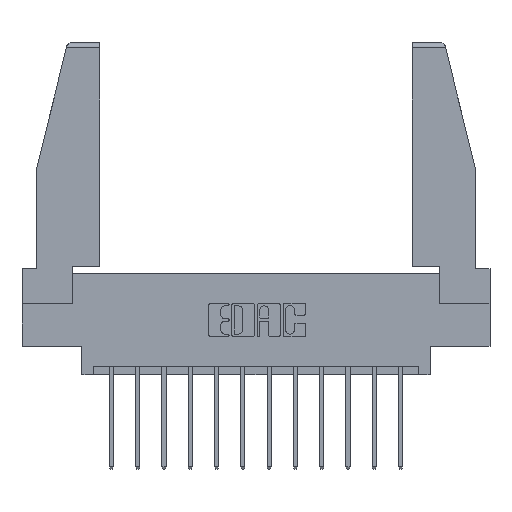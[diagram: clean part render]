
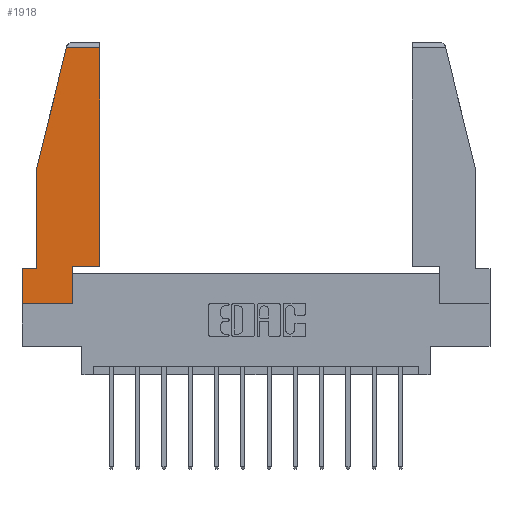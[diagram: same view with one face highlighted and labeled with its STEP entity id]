
A CAD part, top view. The second image highlights one B-rep face of the part: STEP entity #1918.
In plain terms, the highlighted planar face has unit normal (0, 0, 1).
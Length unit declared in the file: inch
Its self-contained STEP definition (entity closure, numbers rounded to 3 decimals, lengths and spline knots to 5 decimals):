
#11 = EDGE_CURVE ( 'NONE', #9317, #4856, #13222, .T. ) ;
#448 = VECTOR ( 'NONE', #8510, 39.37008 ) ;
#564 = VECTOR ( 'NONE', #9412, 39.37008 ) ;
#586 = DIRECTION ( 'NONE',  ( 1., 0., 0. ) ) ;
#639 = DIRECTION ( 'NONE',  ( 1., 0., 0. ) ) ;
#759 = CARTESIAN_POINT ( 'NONE',  ( 0., 1.52, 0. ) ) ;
#765 = VECTOR ( 'NONE', #3878, 39.37008 ) ;
#871 = ORIENTED_EDGE ( 'NONE', *, *, #11598, .T. ) ;
#887 = CARTESIAN_POINT ( 'NONE',  ( 0.297, 0., 0. ) ) ;
#981 = ORIENTED_EDGE ( 'NONE', *, *, #7468, .T. ) ;
#1092 = DIRECTION ( 'NONE',  ( 0., 1., 0. ) ) ;
#1780 = VECTOR ( 'NONE', #6536, 39.37008 ) ;
#1855 = LINE ( 'NONE', #9011, #7597 ) ;
#1918 = ADVANCED_FACE ( 'NONE', ( #15102 ), #10439, .T. ) ;
#2151 = LINE ( 'NONE', #12695, #1780 ) ;
#2437 = ORIENTED_EDGE ( 'NONE', *, *, #12441, .T. ) ;
#2641 = CARTESIAN_POINT ( 'NONE',  ( 0.086, 0.8, 0. ) ) ;
#2787 = VERTEX_POINT ( 'NONE', #12084 ) ;
#2929 = LINE ( 'NONE', #759, #448 ) ;
#3044 = CARTESIAN_POINT ( 'NONE',  ( 0.297, 0.223, 0. ) ) ;
#3161 = EDGE_CURVE ( 'NONE', #2787, #10127, #13903, .T. ) ;
#3176 = LINE ( 'NONE', #12828, #12902 ) ;
#3314 = VERTEX_POINT ( 'NONE', #3661 ) ;
#3504 = VERTEX_POINT ( 'NONE', #10144 ) ;
#3586 = EDGE_LOOP ( 'NONE', ( #15508, #981, #15374, #8361, #9837, #2437, #6179, #11562, #871 ) ) ;
#3661 = CARTESIAN_POINT ( 'NONE',  ( 0.086, 0.21, 0. ) ) ;
#3878 = DIRECTION ( 'NONE',  ( -0.239, -0.971, 0. ) ) ;
#3914 = CARTESIAN_POINT ( 'NONE',  ( 0.461, 0.223, 0. ) ) ;
#4030 = LINE ( 'NONE', #8741, #765 ) ;
#4105 = VERTEX_POINT ( 'NONE', #6369 ) ;
#4177 = EDGE_CURVE ( 'NONE', #4105, #3314, #7805, .T. ) ;
#4770 = CARTESIAN_POINT ( 'NONE',  ( 0.461, 0.223, 0. ) ) ;
#4856 = VERTEX_POINT ( 'NONE', #8624 ) ;
#6179 = ORIENTED_EDGE ( 'NONE', *, *, #12522, .T. ) ;
#6369 = CARTESIAN_POINT ( 'NONE',  ( 0.086, 0.8, 0. ) ) ;
#6416 = CARTESIAN_POINT ( 'NONE',  ( 0., 0., 0. ) ) ;
#6536 = DIRECTION ( 'NONE',  ( -1., 0., 0. ) ) ;
#7234 = VECTOR ( 'NONE', #639, 39.37008 ) ;
#7468 = EDGE_CURVE ( 'NONE', #4856, #12245, #2929, .T. ) ;
#7597 = VECTOR ( 'NONE', #586, 39.37008 ) ;
#7678 = EDGE_CURVE ( 'NONE', #3314, #3504, #2151, .T. ) ;
#7805 = LINE ( 'NONE', #2641, #15059 ) ;
#7808 = DIRECTION ( 'NONE',  ( 0., -1., 0. ) ) ;
#8361 = ORIENTED_EDGE ( 'NONE', *, *, #4177, .T. ) ;
#8510 = DIRECTION ( 'NONE',  ( -1., 0., 0. ) ) ;
#8624 = CARTESIAN_POINT ( 'NONE',  ( 0.461, 1.52, 0. ) ) ;
#8741 = CARTESIAN_POINT ( 'NONE',  ( 0.271, 1.55, 0. ) ) ;
#8818 = EDGE_CURVE ( 'NONE', #12245, #4105, #4030, .T. ) ;
#8999 = CARTESIAN_POINT ( 'NONE',  ( 0., 0., 0. ) ) ;
#9011 = CARTESIAN_POINT ( 'NONE',  ( 0., 0., 0. ) ) ;
#9292 = VERTEX_POINT ( 'NONE', #6416 ) ;
#9317 = VERTEX_POINT ( 'NONE', #3914 ) ;
#9392 = AXIS2_PLACEMENT_3D ( 'NONE', #8999, #13897, #14054 ) ;
#9412 = DIRECTION ( 'NONE',  ( 0., 1., 0. ) ) ;
#9837 = ORIENTED_EDGE ( 'NONE', *, *, #7678, .T. ) ;
#9877 = CARTESIAN_POINT ( 'NONE',  ( 0.2636, 1.52, 0. ) ) ;
#10127 = VERTEX_POINT ( 'NONE', #10152 ) ;
#10144 = CARTESIAN_POINT ( 'NONE',  ( 0., 0.21, 0. ) ) ;
#10152 = CARTESIAN_POINT ( 'NONE',  ( 0.297, 0.223, 0. ) ) ;
#10439 = PLANE ( 'NONE',  #9392 ) ;
#11096 = DIRECTION ( 'NONE',  ( 0., -1., 0. ) ) ;
#11562 = ORIENTED_EDGE ( 'NONE', *, *, #3161, .T. ) ;
#11598 = EDGE_CURVE ( 'NONE', #10127, #9317, #13710, .T. ) ;
#11682 = VECTOR ( 'NONE', #1092, 39.37008 ) ;
#12084 = CARTESIAN_POINT ( 'NONE',  ( 0.297, 0., 0. ) ) ;
#12245 = VERTEX_POINT ( 'NONE', #9877 ) ;
#12441 = EDGE_CURVE ( 'NONE', #3504, #9292, #3176, .T. ) ;
#12522 = EDGE_CURVE ( 'NONE', #9292, #2787, #1855, .T. ) ;
#12695 = CARTESIAN_POINT ( 'NONE',  ( 0., 0.21, 0. ) ) ;
#12828 = CARTESIAN_POINT ( 'NONE',  ( 0., 0.21, 0. ) ) ;
#12902 = VECTOR ( 'NONE', #7808, 39.37008 ) ;
#13222 = LINE ( 'NONE', #4770, #11682 ) ;
#13710 = LINE ( 'NONE', #3044, #7234 ) ;
#13897 = DIRECTION ( 'NONE',  ( 0., 0., 1. ) ) ;
#13903 = LINE ( 'NONE', #887, #564 ) ;
#14054 = DIRECTION ( 'NONE',  ( 1., 0., 0. ) ) ;
#15059 = VECTOR ( 'NONE', #11096, 39.37008 ) ;
#15102 = FACE_OUTER_BOUND ( 'NONE', #3586, .T. ) ;
#15374 = ORIENTED_EDGE ( 'NONE', *, *, #8818, .T. ) ;
#15508 = ORIENTED_EDGE ( 'NONE', *, *, #11, .T. ) ;
